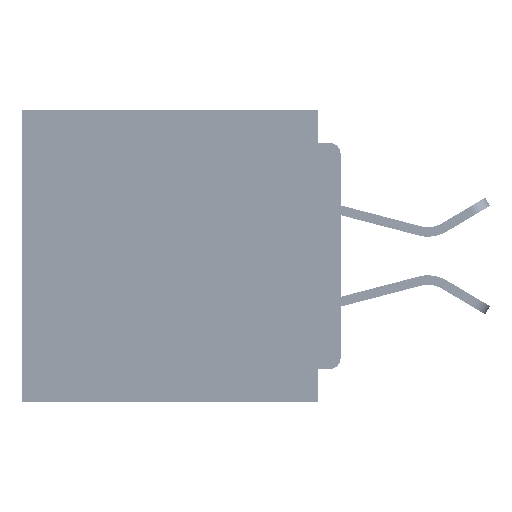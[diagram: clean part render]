
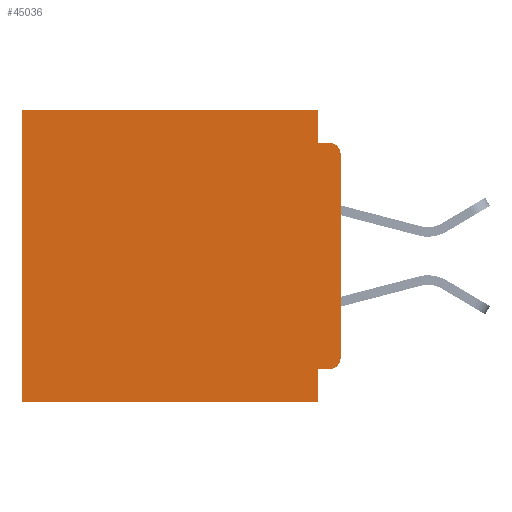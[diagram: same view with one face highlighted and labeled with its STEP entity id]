
A CAD part, left-side view. The second image highlights one B-rep face of the part: STEP entity #45036.
In plain terms, the highlighted planar face has unit normal (-1, 0, 0).
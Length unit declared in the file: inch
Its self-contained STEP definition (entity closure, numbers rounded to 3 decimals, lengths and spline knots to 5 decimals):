
#45 = VERTEX_POINT ( 'NONE', #44354 ) ;
#48 = LINE ( 'NONE', #24692, #23639 ) ;
#87 = ORIENTED_EDGE ( 'NONE', *, *, #32267, .T. ) ;
#738 = DIRECTION ( 'NONE',  ( -1., 0., 0. ) ) ;
#2691 = VECTOR ( 'NONE', #18258, 39.37008 ) ;
#2978 = CARTESIAN_POINT ( 'NONE',  ( 0.3, 0.031, -0.4 ) ) ;
#4013 = DIRECTION ( 'NONE',  ( 0., 0., -1. ) ) ;
#4036 = CARTESIAN_POINT ( 'NONE',  ( 0.3, 0.015, -0.06 ) ) ;
#4234 = EDGE_CURVE ( 'NONE', #45, #29005, #23644, .T. ) ;
#5618 = EDGE_CURVE ( 'NONE', #58429, #45, #56997, .T. ) ;
#6115 = CARTESIAN_POINT ( 'NONE',  ( 0.3, 0., 0. ) ) ;
#6123 = LINE ( 'NONE', #6115, #54525 ) ;
#6450 = DIRECTION ( 'NONE',  ( 0., 0., -1. ) ) ;
#7243 = DIRECTION ( 'NONE',  ( 1., 0., 0. ) ) ;
#8735 = CIRCLE ( 'NONE', #50605, 0.015 ) ;
#8782 = DIRECTION ( 'NONE',  ( 0., 0., -1. ) ) ;
#9830 = ORIENTED_EDGE ( 'NONE', *, *, #5618, .F. ) ;
#10128 = ORIENTED_EDGE ( 'NONE', *, *, #54071, .F. ) ;
#10839 = DIRECTION ( 'NONE',  ( 0., 1., 0. ) ) ;
#10893 = EDGE_CURVE ( 'NONE', #58429, #51465, #8735, .T. ) ;
#11117 = VECTOR ( 'NONE', #4013, 39.37008 ) ;
#13535 = CARTESIAN_POINT ( 'NONE',  ( 0.3, 0., -0.4 ) ) ;
#13936 = LINE ( 'NONE', #50505, #49860 ) ;
#14507 = VECTOR ( 'NONE', #24076, 39.37008 ) ;
#15589 = ORIENTED_EDGE ( 'NONE', *, *, #48328, .F. ) ;
#15969 = CARTESIAN_POINT ( 'NONE',  ( 0.3, 0.437, -0.4 ) ) ;
#17166 = VECTOR ( 'NONE', #6450, 39.37008 ) ;
#18258 = DIRECTION ( 'NONE',  ( 0., 1., 0. ) ) ;
#18672 = LINE ( 'NONE', #43981, #17166 ) ;
#19349 = CARTESIAN_POINT ( 'NONE',  ( 0.3, 0., -0.045 ) ) ;
#19517 = CARTESIAN_POINT ( 'NONE',  ( 0.3, 0., -0.06 ) ) ;
#20713 = EDGE_CURVE ( 'NONE', #44177, #51465, #48, .T. ) ;
#20895 = AXIS2_PLACEMENT_3D ( 'NONE', #4036, #36975, #8782 ) ;
#21146 = VECTOR ( 'NONE', #59673, 39.37008 ) ;
#21903 = EDGE_LOOP ( 'NONE', ( #52005, #87, #15589, #42253, #42432, #44077, #10128, #41396, #9830, #51045 ) ) ;
#22604 = CARTESIAN_POINT ( 'NONE',  ( 0.3, 0., -0.34 ) ) ;
#23639 = VECTOR ( 'NONE', #29440, 39.37008 ) ;
#23644 = LINE ( 'NONE', #2978, #11117 ) ;
#23780 = AXIS2_PLACEMENT_3D ( 'NONE', #58654, #7243, #40113 ) ;
#24076 = DIRECTION ( 'NONE',  ( 0., -1., 0. ) ) ;
#24692 = CARTESIAN_POINT ( 'NONE',  ( 0.3, 0., -0.4 ) ) ;
#25860 = EDGE_CURVE ( 'NONE', #34683, #44314, #18672, .T. ) ;
#26455 = CIRCLE ( 'NONE', #20895, 0.015 ) ;
#28980 = CARTESIAN_POINT ( 'NONE',  ( 0.3, 0.015, -0.34 ) ) ;
#29005 = VERTEX_POINT ( 'NONE', #55561 ) ;
#29440 = DIRECTION ( 'NONE',  ( 0., 0., -1. ) ) ;
#31577 = EDGE_CURVE ( 'NONE', #50169, #36846, #13936, .T. ) ;
#32267 = EDGE_CURVE ( 'NONE', #44177, #41065, #26455, .T. ) ;
#33344 = CARTESIAN_POINT ( 'NONE',  ( 0.3, 0.031, 0. ) ) ;
#33707 = DIRECTION ( 'NONE',  ( 0., 0., -1. ) ) ;
#34000 = FACE_OUTER_BOUND ( 'NONE', #21903, .T. ) ;
#34683 = VERTEX_POINT ( 'NONE', #56613 ) ;
#35443 = PLANE ( 'NONE',  #23780 ) ;
#36642 = DIRECTION ( 'NONE',  ( 0., 0., -1. ) ) ;
#36846 = VERTEX_POINT ( 'NONE', #40166 ) ;
#36975 = DIRECTION ( 'NONE',  ( -1., 0., 0. ) ) ;
#40113 = DIRECTION ( 'NONE',  ( 0., 0., -1. ) ) ;
#40166 = CARTESIAN_POINT ( 'NONE',  ( 0.3, 0.031, -0.045 ) ) ;
#41065 = VERTEX_POINT ( 'NONE', #41945 ) ;
#41396 = ORIENTED_EDGE ( 'NONE', *, *, #4234, .F. ) ;
#41945 = CARTESIAN_POINT ( 'NONE',  ( 0.3, 0.015, -0.045 ) ) ;
#42253 = ORIENTED_EDGE ( 'NONE', *, *, #31577, .F. ) ;
#42432 = ORIENTED_EDGE ( 'NONE', *, *, #44272, .T. ) ;
#43981 = CARTESIAN_POINT ( 'NONE',  ( 0.3, 0.437, -0.4 ) ) ;
#44077 = ORIENTED_EDGE ( 'NONE', *, *, #25860, .T. ) ;
#44177 = VERTEX_POINT ( 'NONE', #19517 ) ;
#44272 = EDGE_CURVE ( 'NONE', #50169, #34683, #6123, .T. ) ;
#44314 = VERTEX_POINT ( 'NONE', #15969 ) ;
#44354 = CARTESIAN_POINT ( 'NONE',  ( 0.3, 0.031, -0.355 ) ) ;
#45036 = ADVANCED_FACE ( 'NONE', ( #34000 ), #35443, .F. ) ;
#45806 = CARTESIAN_POINT ( 'NONE',  ( 0.3, 0., -0.355 ) ) ;
#48328 = EDGE_CURVE ( 'NONE', #36846, #41065, #48975, .T. ) ;
#48975 = LINE ( 'NONE', #19349, #14507 ) ;
#49860 = VECTOR ( 'NONE', #36642, 39.37008 ) ;
#50169 = VERTEX_POINT ( 'NONE', #33344 ) ;
#50505 = CARTESIAN_POINT ( 'NONE',  ( 0.3, 0.031, 0. ) ) ;
#50605 = AXIS2_PLACEMENT_3D ( 'NONE', #28980, #738, #33707 ) ;
#51045 = ORIENTED_EDGE ( 'NONE', *, *, #10893, .T. ) ;
#51465 = VERTEX_POINT ( 'NONE', #22604 ) ;
#52005 = ORIENTED_EDGE ( 'NONE', *, *, #20713, .F. ) ;
#52625 = LINE ( 'NONE', #13535, #2691 ) ;
#54071 = EDGE_CURVE ( 'NONE', #29005, #44314, #52625, .T. ) ;
#54525 = VECTOR ( 'NONE', #10839, 39.37008 ) ;
#55561 = CARTESIAN_POINT ( 'NONE',  ( 0.3, 0.031, -0.4 ) ) ;
#56613 = CARTESIAN_POINT ( 'NONE',  ( 0.3, 0.437, 0. ) ) ;
#56997 = LINE ( 'NONE', #45806, #21146 ) ;
#57067 = CARTESIAN_POINT ( 'NONE',  ( 0.3, 0.015, -0.355 ) ) ;
#58429 = VERTEX_POINT ( 'NONE', #57067 ) ;
#58654 = CARTESIAN_POINT ( 'NONE',  ( 0.3, 0., -0.4 ) ) ;
#59673 = DIRECTION ( 'NONE',  ( 0., 1., 0. ) ) ;
